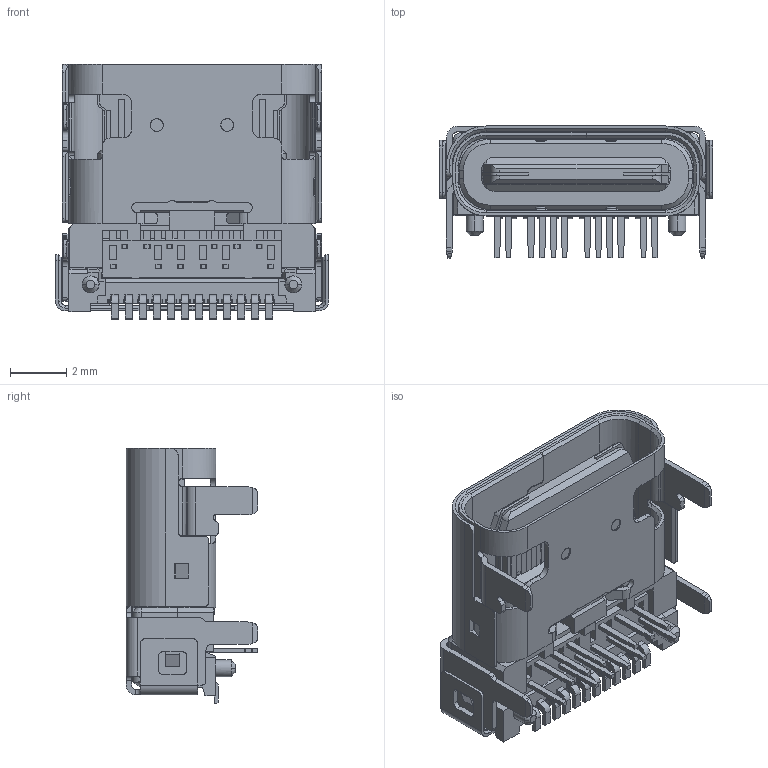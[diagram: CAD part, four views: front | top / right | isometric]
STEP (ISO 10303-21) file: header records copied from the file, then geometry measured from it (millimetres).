
FILE_DESCRIPTION (( 'STEP AP214' ), '1' );
FILE_NAME ('698C124-206-211.STEP', '2021-01-15T18:06:15', ( '' ), ( '' ), 'SwSTEP 2.0', 'SolidWorks 2020', '' );
FILE_SCHEMA (( 'AUTOMOTIVE_DESIGN' ));
Length unit declared in the file: millimetre
Products named in the file (3): 698C124-206-211; Shell 698C124-X06-211; Insulator 698C124-X06-211
Assembly tree (2 placements, depth 2):
  698C124-206-211
    Shell 698C124-X06-211
    Insulator 698C124-X06-211
Bounding box: 9.7 x 4.68 x 9.06 mm (x, y, z)
Volume: 146.2 mm3; surface area: 931.2 mm2
Topology: 2 solids, 2 shells, 2101 faces, 6181 edges, 4091 vertices
Faces by surface type: plane 1490, cylinder 537, cone 56, bspline 18
Entity records: 77230 total; most frequent: CARTESIAN_POINT 19457, ORIENTED_EDGE 12362, DIRECTION 9242, EDGE_CURVE 6181, VECTOR 4200, LINE 4200, VERTEX_POINT 4091, AXIS2_PLACEMENT_3D 2521
